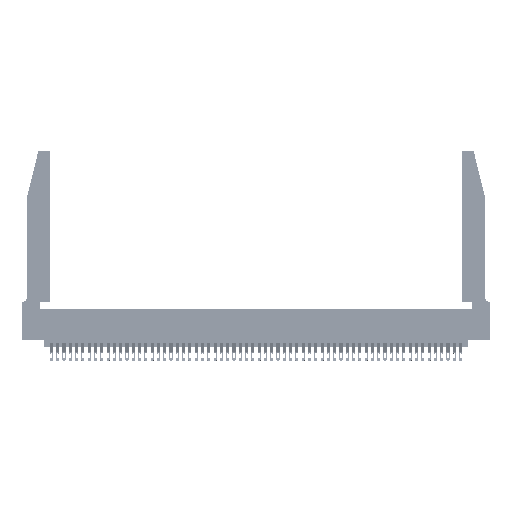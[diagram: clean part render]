
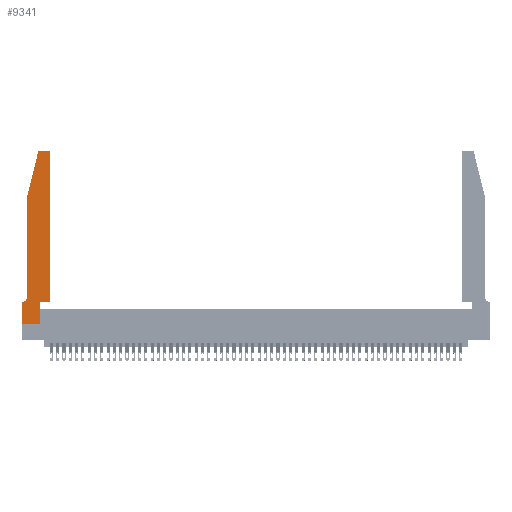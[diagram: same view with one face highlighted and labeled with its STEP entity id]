
A CAD part, top view. The second image highlights one B-rep face of the part: STEP entity #9341.
In plain terms, the highlighted planar face has unit normal (0, 0, 1).
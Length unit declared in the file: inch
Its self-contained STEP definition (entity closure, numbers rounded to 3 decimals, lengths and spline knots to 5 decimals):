
#58 = EDGE_CURVE ( 'NONE', #32030, #29689, #7124, .T. ) ;
#488 = EDGE_CURVE ( 'NONE', #13761, #38833, #8326, .T. ) ;
#1031 = PLANE ( 'NONE',  #21850 ) ;
#2113 = ORIENTED_EDGE ( 'NONE', *, *, #25463, .T. ) ;
#2813 = FACE_OUTER_BOUND ( 'NONE', #27878, .T. ) ;
#2997 = VECTOR ( 'NONE', #10579, 39.37008 ) ;
#3724 = LINE ( 'NONE', #32435, #49202 ) ;
#4240 = VECTOR ( 'NONE', #9157, 39.37008 ) ;
#4938 = DIRECTION ( 'NONE',  ( -1., 0., 0. ) ) ;
#5078 = CARTESIAN_POINT ( 'NONE',  ( 0.4505, 2.72, 0.37 ) ) ;
#5265 = CIRCLE ( 'NONE', #24640, 0.03 ) ;
#5607 = ORIENTED_EDGE ( 'NONE', *, *, #12537, .T. ) ;
#7124 = LINE ( 'NONE', #36236, #36317 ) ;
#7634 = VECTOR ( 'NONE', #4938, 39.37008 ) ;
#8245 = VECTOR ( 'NONE', #52875, 39.37008 ) ;
#8326 = LINE ( 'NONE', #16026, #36262 ) ;
#9157 = DIRECTION ( 'NONE',  ( 0., 1., 0. ) ) ;
#9341 = ADVANCED_FACE ( 'NONE', ( #2813 ), #1031, .T. ) ;
#9420 = ORIENTED_EDGE ( 'NONE', *, *, #30542, .T. ) ;
#10293 = CIRCLE ( 'NONE', #17442, 0.07 ) ;
#10579 = DIRECTION ( 'NONE',  ( -1., 0., 0. ) ) ;
#11296 = DIRECTION ( 'NONE',  ( 1., 0., 0. ) ) ;
#11367 = DIRECTION ( 'NONE',  ( 0., 1., 0. ) ) ;
#12537 = EDGE_CURVE ( 'NONE', #29689, #45851, #3724, .T. ) ;
#13761 = VERTEX_POINT ( 'NONE', #20356 ) ;
#15091 = CARTESIAN_POINT ( 'NONE',  ( 0.25487, 2.72718, 0.37 ) ) ;
#15371 = CARTESIAN_POINT ( 'NONE',  ( 0.0755, 0.42, 0.37 ) ) ;
#15431 = VERTEX_POINT ( 'NONE', #18574 ) ;
#15955 = DIRECTION ( 'NONE',  ( 1., 0., 0. ) ) ;
#16026 = CARTESIAN_POINT ( 'NONE',  ( 0.0755, 2., 0.37 ) ) ;
#16190 = VERTEX_POINT ( 'NONE', #47756 ) ;
#17113 = CIRCLE ( 'NONE', #34333, 0.03 ) ;
#17442 = AXIS2_PLACEMENT_3D ( 'NONE', #44579, #23172, #48766 ) ;
#17708 = DIRECTION ( 'NONE',  ( 0., 0., 1. ) ) ;
#18574 = CARTESIAN_POINT ( 'NONE',  ( 0.284, 2.75, 0.37 ) ) ;
#19836 = CARTESIAN_POINT ( 'NONE',  ( 0., 0., 0.37 ) ) ;
#19944 = DIRECTION ( 'NONE',  ( 0., 0., 1. ) ) ;
#20356 = CARTESIAN_POINT ( 'NONE',  ( 0.0755, 2., 0.37 ) ) ;
#21798 = ORIENTED_EDGE ( 'NONE', *, *, #28265, .T. ) ;
#21850 = AXIS2_PLACEMENT_3D ( 'NONE', #30070, #17708, #38620 ) ;
#22566 = VERTEX_POINT ( 'NONE', #44622 ) ;
#23172 = DIRECTION ( 'NONE',  ( 0., 0., -1. ) ) ;
#24638 = CARTESIAN_POINT ( 'NONE',  ( 0.4505, 0.35, 0.37 ) ) ;
#24640 = AXIS2_PLACEMENT_3D ( 'NONE', #41023, #19944, #15955 ) ;
#25382 = CARTESIAN_POINT ( 'NONE',  ( 0.0755, 2., 0.37 ) ) ;
#25463 = EDGE_CURVE ( 'NONE', #16190, #22566, #40786, .T. ) ;
#25550 = DIRECTION ( 'NONE',  ( -0.239, -0.971, 0. ) ) ;
#25679 = CARTESIAN_POINT ( 'NONE',  ( 0.2605, 2.75, 0.37 ) ) ;
#26377 = CARTESIAN_POINT ( 'NONE',  ( 0.4505, 0.35, 0.37 ) ) ;
#27878 = EDGE_LOOP ( 'NONE', ( #29627, #49026, #21798, #40097, #9420, #31427, #2113, #47251, #50686, #5607, #51271, #47943 ) ) ;
#28265 = EDGE_CURVE ( 'NONE', #31264, #13761, #30681, .T. ) ;
#28372 = DIRECTION ( 'NONE',  ( 0., -1., 0. ) ) ;
#29330 = CARTESIAN_POINT ( 'NONE',  ( 0.2865, 0., 0.37 ) ) ;
#29556 = LINE ( 'NONE', #24638, #4240 ) ;
#29627 = ORIENTED_EDGE ( 'NONE', *, *, #30841, .T. ) ;
#29689 = VERTEX_POINT ( 'NONE', #33930 ) ;
#30070 = CARTESIAN_POINT ( 'NONE',  ( 0., 0.35, 0.37 ) ) ;
#30542 = EDGE_CURVE ( 'NONE', #38833, #30608, #10293, .T. ) ;
#30608 = VERTEX_POINT ( 'NONE', #35862 ) ;
#30681 = LINE ( 'NONE', #25382, #35265 ) ;
#30841 = EDGE_CURVE ( 'NONE', #42684, #15431, #42063, .T. ) ;
#31027 = LINE ( 'NONE', #36316, #8245 ) ;
#31264 = VERTEX_POINT ( 'NONE', #15091 ) ;
#31427 = ORIENTED_EDGE ( 'NONE', *, *, #46520, .T. ) ;
#32030 = VERTEX_POINT ( 'NONE', #29330 ) ;
#32090 = EDGE_CURVE ( 'NONE', #45851, #45666, #29556, .T. ) ;
#32435 = CARTESIAN_POINT ( 'NONE',  ( 0.4505, 0.35, 0.37 ) ) ;
#33930 = CARTESIAN_POINT ( 'NONE',  ( 0.2865, 0.35, 0.37 ) ) ;
#34333 = AXIS2_PLACEMENT_3D ( 'NONE', #40886, #48540, #11296 ) ;
#35265 = VECTOR ( 'NONE', #25550, 39.37008 ) ;
#35862 = CARTESIAN_POINT ( 'NONE',  ( 0.0055, 0.35, 0.37 ) ) ;
#36236 = CARTESIAN_POINT ( 'NONE',  ( 0.2865, 0.35, 0.37 ) ) ;
#36262 = VECTOR ( 'NONE', #43063, 39.37008 ) ;
#36316 = CARTESIAN_POINT ( 'NONE',  ( 0., 0., 0.37 ) ) ;
#36317 = VECTOR ( 'NONE', #11367, 39.37008 ) ;
#36957 = EDGE_CURVE ( 'NONE', #15431, #31264, #5265, .T. ) ;
#37548 = VECTOR ( 'NONE', #28372, 39.37008 ) ;
#38620 = DIRECTION ( 'NONE',  ( 1., 0., 0. ) ) ;
#38833 = VERTEX_POINT ( 'NONE', #15371 ) ;
#39841 = EDGE_CURVE ( 'NONE', #22566, #32030, #31027, .T. ) ;
#40097 = ORIENTED_EDGE ( 'NONE', *, *, #488, .T. ) ;
#40786 = LINE ( 'NONE', #19836, #37548 ) ;
#40886 = CARTESIAN_POINT ( 'NONE',  ( 0.4205, 2.72, 0.37 ) ) ;
#41023 = CARTESIAN_POINT ( 'NONE',  ( 0.284, 2.72, 0.37 ) ) ;
#42063 = LINE ( 'NONE', #25679, #7634 ) ;
#42684 = VERTEX_POINT ( 'NONE', #44631 ) ;
#43063 = DIRECTION ( 'NONE',  ( 0., -1., 0. ) ) ;
#43994 = CARTESIAN_POINT ( 'NONE',  ( 0.0755, 0.35, 0.37 ) ) ;
#44579 = CARTESIAN_POINT ( 'NONE',  ( 0.0055, 0.42, 0.37 ) ) ;
#44622 = CARTESIAN_POINT ( 'NONE',  ( 0., 0., 0.37 ) ) ;
#44631 = CARTESIAN_POINT ( 'NONE',  ( 0.4205, 2.75, 0.37 ) ) ;
#45666 = VERTEX_POINT ( 'NONE', #5078 ) ;
#45851 = VERTEX_POINT ( 'NONE', #26377 ) ;
#46520 = EDGE_CURVE ( 'NONE', #30608, #16190, #51133, .T. ) ;
#47251 = ORIENTED_EDGE ( 'NONE', *, *, #39841, .T. ) ;
#47756 = CARTESIAN_POINT ( 'NONE',  ( 0., 0.35, 0.37 ) ) ;
#47943 = ORIENTED_EDGE ( 'NONE', *, *, #48017, .T. ) ;
#48017 = EDGE_CURVE ( 'NONE', #45666, #42684, #17113, .T. ) ;
#48540 = DIRECTION ( 'NONE',  ( 0., 0., 1. ) ) ;
#48766 = DIRECTION ( 'NONE',  ( -1., 0., 0. ) ) ;
#49026 = ORIENTED_EDGE ( 'NONE', *, *, #36957, .T. ) ;
#49202 = VECTOR ( 'NONE', #53490, 39.37008 ) ;
#50686 = ORIENTED_EDGE ( 'NONE', *, *, #58, .T. ) ;
#51133 = LINE ( 'NONE', #43994, #2997 ) ;
#51271 = ORIENTED_EDGE ( 'NONE', *, *, #32090, .T. ) ;
#52875 = DIRECTION ( 'NONE',  ( 1., 0., 0. ) ) ;
#53490 = DIRECTION ( 'NONE',  ( 1., 0., 0. ) ) ;
